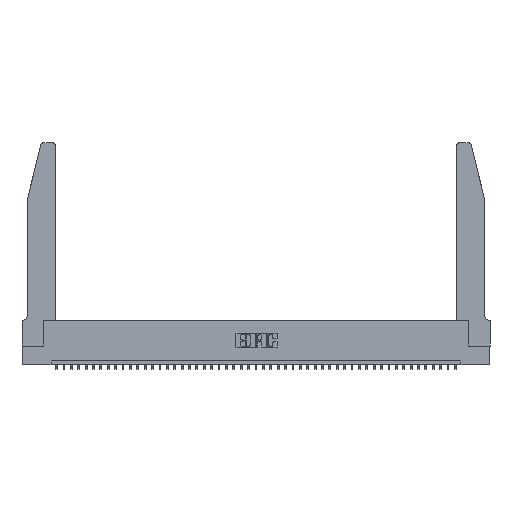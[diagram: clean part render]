
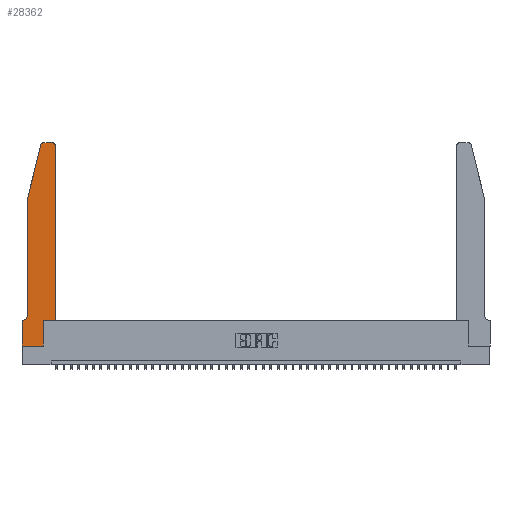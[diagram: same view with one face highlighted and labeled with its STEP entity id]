
A CAD part, top view. The second image highlights one B-rep face of the part: STEP entity #28362.
In plain terms, the highlighted planar face has unit normal (0, 0, 1).
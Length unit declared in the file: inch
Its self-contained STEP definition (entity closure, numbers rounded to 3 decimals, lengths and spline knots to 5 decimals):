
#922 = CARTESIAN_POINT ( 'NONE',  ( 0.0755, 2., 0.37 ) ) ;
#1184 = VERTEX_POINT ( 'NONE', #12597 ) ;
#1337 = CARTESIAN_POINT ( 'NONE',  ( 0.4205, 2.72, 0.37 ) ) ;
#1771 = VERTEX_POINT ( 'NONE', #5098 ) ;
#3221 = EDGE_CURVE ( 'NONE', #7878, #14248, #22996, .T. ) ;
#3448 = CIRCLE ( 'NONE', #18407, 0.07 ) ;
#3516 = PLANE ( 'NONE',  #17269 ) ;
#3671 = DIRECTION ( 'NONE',  ( 0., 0., 1. ) ) ;
#3841 = ORIENTED_EDGE ( 'NONE', *, *, #21381, .T. ) ;
#4326 = EDGE_CURVE ( 'NONE', #44307, #14060, #3448, .T. ) ;
#4558 = DIRECTION ( 'NONE',  ( -0.239, -0.971, 0. ) ) ;
#5098 = CARTESIAN_POINT ( 'NONE',  ( 0.4505, 0.35, 0.37 ) ) ;
#5196 = DIRECTION ( 'NONE',  ( -1., 0., 0. ) ) ;
#5227 = VERTEX_POINT ( 'NONE', #44248 ) ;
#5294 = CARTESIAN_POINT ( 'NONE',  ( 0.0755, 0.42, 0.37 ) ) ;
#5487 = CARTESIAN_POINT ( 'NONE',  ( 0.4505, 2.72, 0.37 ) ) ;
#6234 = DIRECTION ( 'NONE',  ( 0., 1., 0. ) ) ;
#6776 = ORIENTED_EDGE ( 'NONE', *, *, #26556, .T. ) ;
#7878 = VERTEX_POINT ( 'NONE', #17926 ) ;
#8062 = VECTOR ( 'NONE', #39020, 39.37008 ) ;
#8336 = FACE_OUTER_BOUND ( 'NONE', #18337, .T. ) ;
#8460 = LINE ( 'NONE', #43027, #18238 ) ;
#9365 = CARTESIAN_POINT ( 'NONE',  ( 0.4505, 0.35, 0.37 ) ) ;
#9957 = EDGE_CURVE ( 'NONE', #25072, #5227, #8460, .T. ) ;
#10073 = VECTOR ( 'NONE', #6234, 39.37008 ) ;
#10135 = VECTOR ( 'NONE', #5196, 39.37008 ) ;
#10342 = VERTEX_POINT ( 'NONE', #30658 ) ;
#10534 = CARTESIAN_POINT ( 'NONE',  ( 0., 0., 0.37 ) ) ;
#10602 = DIRECTION ( 'NONE',  ( 1., 0., 0. ) ) ;
#10712 = VERTEX_POINT ( 'NONE', #39066 ) ;
#11094 = ORIENTED_EDGE ( 'NONE', *, *, #28954, .T. ) ;
#11510 = VECTOR ( 'NONE', #37225, 39.37008 ) ;
#11613 = CARTESIAN_POINT ( 'NONE',  ( 0.0055, 0.35, 0.37 ) ) ;
#11719 = LINE ( 'NONE', #43186, #10135 ) ;
#12597 = CARTESIAN_POINT ( 'NONE',  ( 0., 0., 0.37 ) ) ;
#14060 = VERTEX_POINT ( 'NONE', #11613 ) ;
#14248 = VERTEX_POINT ( 'NONE', #20833 ) ;
#15538 = VECTOR ( 'NONE', #4558, 39.37008 ) ;
#16340 = CARTESIAN_POINT ( 'NONE',  ( 0.284, 2.72, 0.37 ) ) ;
#17202 = DIRECTION ( 'NONE',  ( 1., 0., 0. ) ) ;
#17269 = AXIS2_PLACEMENT_3D ( 'NONE', #31130, #3671, #10602 ) ;
#17286 = LINE ( 'NONE', #9365, #43532 ) ;
#17652 = CIRCLE ( 'NONE', #24777, 0.03 ) ;
#17926 = CARTESIAN_POINT ( 'NONE',  ( 0.2865, 0., 0.37 ) ) ;
#18124 = VERTEX_POINT ( 'NONE', #32510 ) ;
#18238 = VECTOR ( 'NONE', #32766, 39.37008 ) ;
#18337 = EDGE_LOOP ( 'NONE', ( #23565, #26231, #6776, #41095, #30016, #30287, #26943, #43809, #19207, #3841, #41172, #11094 ) ) ;
#18407 = AXIS2_PLACEMENT_3D ( 'NONE', #24227, #27708, #23939 ) ;
#18853 = VERTEX_POINT ( 'NONE', #5487 ) ;
#19207 = ORIENTED_EDGE ( 'NONE', *, *, #3221, .T. ) ;
#19956 = CARTESIAN_POINT ( 'NONE',  ( 0.4205, 2.75, 0.37 ) ) ;
#20429 = LINE ( 'NONE', #10534, #21505 ) ;
#20833 = CARTESIAN_POINT ( 'NONE',  ( 0.2865, 0.35, 0.37 ) ) ;
#21254 = AXIS2_PLACEMENT_3D ( 'NONE', #16340, #30085, #40319 ) ;
#21381 = EDGE_CURVE ( 'NONE', #14248, #1771, #35567, .T. ) ;
#21505 = VECTOR ( 'NONE', #17202, 39.37008 ) ;
#21872 = EDGE_CURVE ( 'NONE', #1184, #7878, #20429, .T. ) ;
#22529 = EDGE_CURVE ( 'NONE', #10712, #1184, #38374, .T. ) ;
#22951 = EDGE_CURVE ( 'NONE', #10342, #44307, #40510, .T. ) ;
#22996 = LINE ( 'NONE', #33653, #10073 ) ;
#23565 = ORIENTED_EDGE ( 'NONE', *, *, #9957, .T. ) ;
#23939 = DIRECTION ( 'NONE',  ( -1., 0., 0. ) ) ;
#24227 = CARTESIAN_POINT ( 'NONE',  ( 0.0055, 0.42, 0.37 ) ) ;
#24777 = AXIS2_PLACEMENT_3D ( 'NONE', #1337, #32579, #25499 ) ;
#25072 = VERTEX_POINT ( 'NONE', #19956 ) ;
#25130 = CARTESIAN_POINT ( 'NONE',  ( 0.4505, 0.35, 0.37 ) ) ;
#25499 = DIRECTION ( 'NONE',  ( 1., 0., 0. ) ) ;
#26231 = ORIENTED_EDGE ( 'NONE', *, *, #39384, .T. ) ;
#26556 = EDGE_CURVE ( 'NONE', #18124, #10342, #43417, .T. ) ;
#26943 = ORIENTED_EDGE ( 'NONE', *, *, #22529, .T. ) ;
#27280 = CIRCLE ( 'NONE', #21254, 0.03 ) ;
#27708 = DIRECTION ( 'NONE',  ( 0., 0., -1. ) ) ;
#28362 = ADVANCED_FACE ( 'NONE', ( #8336 ), #3516, .T. ) ;
#28954 = EDGE_CURVE ( 'NONE', #18853, #25072, #17652, .T. ) ;
#29700 = EDGE_CURVE ( 'NONE', #1771, #18853, #17286, .T. ) ;
#30016 = ORIENTED_EDGE ( 'NONE', *, *, #4326, .T. ) ;
#30085 = DIRECTION ( 'NONE',  ( 0., 0., 1. ) ) ;
#30287 = ORIENTED_EDGE ( 'NONE', *, *, #43669, .T. ) ;
#30658 = CARTESIAN_POINT ( 'NONE',  ( 0.0755, 2., 0.37 ) ) ;
#31130 = CARTESIAN_POINT ( 'NONE',  ( 0., 0.35, 0.37 ) ) ;
#32510 = CARTESIAN_POINT ( 'NONE',  ( 0.25487, 2.72718, 0.37 ) ) ;
#32579 = DIRECTION ( 'NONE',  ( 0., 0., 1. ) ) ;
#32766 = DIRECTION ( 'NONE',  ( -1., 0., 0. ) ) ;
#33653 = CARTESIAN_POINT ( 'NONE',  ( 0.2865, 0.35, 0.37 ) ) ;
#35567 = LINE ( 'NONE', #25130, #8062 ) ;
#35782 = VECTOR ( 'NONE', #37298, 39.37008 ) ;
#36864 = DIRECTION ( 'NONE',  ( 0., 1., 0. ) ) ;
#37074 = CARTESIAN_POINT ( 'NONE',  ( 0.0755, 2., 0.37 ) ) ;
#37225 = DIRECTION ( 'NONE',  ( 0., -1., 0. ) ) ;
#37298 = DIRECTION ( 'NONE',  ( 0., -1., 0. ) ) ;
#38374 = LINE ( 'NONE', #44293, #35782 ) ;
#39020 = DIRECTION ( 'NONE',  ( 1., 0., 0. ) ) ;
#39066 = CARTESIAN_POINT ( 'NONE',  ( 0., 0.35, 0.37 ) ) ;
#39384 = EDGE_CURVE ( 'NONE', #5227, #18124, #27280, .T. ) ;
#40319 = DIRECTION ( 'NONE',  ( 1., 0., 0. ) ) ;
#40510 = LINE ( 'NONE', #37074, #11510 ) ;
#41095 = ORIENTED_EDGE ( 'NONE', *, *, #22951, .T. ) ;
#41172 = ORIENTED_EDGE ( 'NONE', *, *, #29700, .T. ) ;
#43027 = CARTESIAN_POINT ( 'NONE',  ( 0.2605, 2.75, 0.37 ) ) ;
#43186 = CARTESIAN_POINT ( 'NONE',  ( 0.0755, 0.35, 0.37 ) ) ;
#43417 = LINE ( 'NONE', #922, #15538 ) ;
#43532 = VECTOR ( 'NONE', #36864, 39.37008 ) ;
#43669 = EDGE_CURVE ( 'NONE', #14060, #10712, #11719, .T. ) ;
#43809 = ORIENTED_EDGE ( 'NONE', *, *, #21872, .T. ) ;
#44248 = CARTESIAN_POINT ( 'NONE',  ( 0.284, 2.75, 0.37 ) ) ;
#44293 = CARTESIAN_POINT ( 'NONE',  ( 0., 0., 0.37 ) ) ;
#44307 = VERTEX_POINT ( 'NONE', #5294 ) ;
